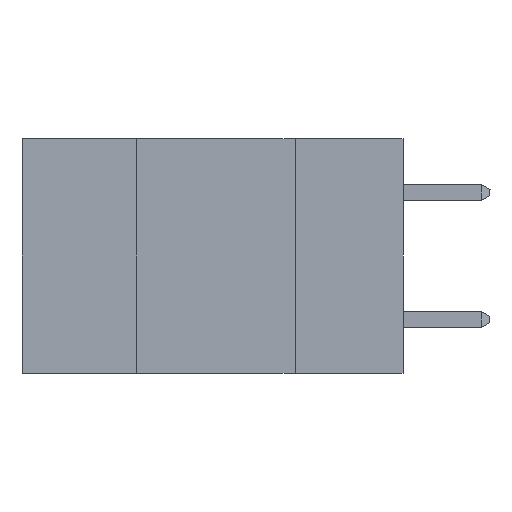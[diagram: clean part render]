
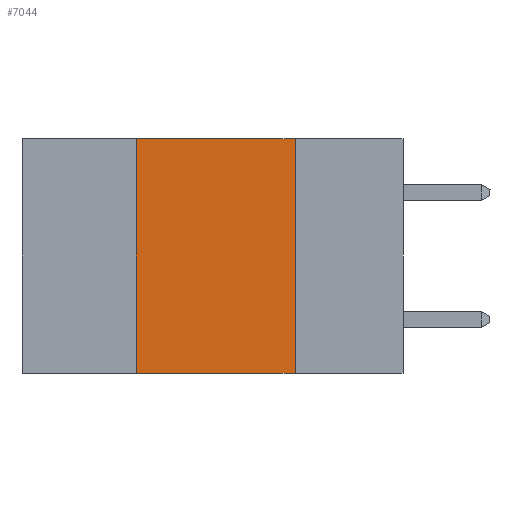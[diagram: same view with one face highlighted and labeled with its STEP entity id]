
A CAD part, left-side view. The second image highlights one B-rep face of the part: STEP entity #7044.
In plain terms, the highlighted planar face has unit normal (-1, 0, 0).
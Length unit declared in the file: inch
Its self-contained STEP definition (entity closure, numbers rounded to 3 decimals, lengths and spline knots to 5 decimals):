
#119 = LINE ( 'NONE', #8788, #1291 ) ;
#154 = CARTESIAN_POINT ( 'NONE',  ( 0., 0.17, -0.37 ) ) ;
#799 = ORIENTED_EDGE ( 'NONE', *, *, #2144, .T. ) ;
#1194 = ORIENTED_EDGE ( 'NONE', *, *, #5678, .F. ) ;
#1291 = VECTOR ( 'NONE', #3387, 39.37008 ) ;
#1504 = LINE ( 'NONE', #10190, #4808 ) ;
#1773 = DIRECTION ( 'NONE',  ( 0., 0., -1. ) ) ;
#2144 = EDGE_CURVE ( 'NONE', #11082, #13219, #7623, .T. ) ;
#2522 = EDGE_LOOP ( 'NONE', ( #8219, #12544, #1194, #799 ) ) ;
#2592 = DIRECTION ( 'NONE',  ( 0., 0., 1. ) ) ;
#2691 = EDGE_CURVE ( 'NONE', #8014, #13219, #1504, .T. ) ;
#3028 = CARTESIAN_POINT ( 'NONE',  ( 0., 0.17, 0. ) ) ;
#3387 = DIRECTION ( 'NONE',  ( 0., -1., 0. ) ) ;
#4664 = CARTESIAN_POINT ( 'NONE',  ( 0., 0.6, 0. ) ) ;
#4808 = VECTOR ( 'NONE', #1773, 39.37008 ) ;
#4813 = LINE ( 'NONE', #5727, #12065 ) ;
#5678 = EDGE_CURVE ( 'NONE', #11082, #12973, #4813, .T. ) ;
#5727 = CARTESIAN_POINT ( 'NONE',  ( 0., 0.42, 0. ) ) ;
#5732 = FACE_OUTER_BOUND ( 'NONE', #2522, .T. ) ;
#6854 = DIRECTION ( 'NONE',  ( 0., -1., 0. ) ) ;
#7044 = ADVANCED_FACE ( 'NONE', ( #5732 ), #10071, .F. ) ;
#7623 = LINE ( 'NONE', #8764, #9974 ) ;
#7770 = CARTESIAN_POINT ( 'NONE',  ( 0., 0.42, 0. ) ) ;
#8014 = VERTEX_POINT ( 'NONE', #3028 ) ;
#8219 = ORIENTED_EDGE ( 'NONE', *, *, #2691, .F. ) ;
#8764 = CARTESIAN_POINT ( 'NONE',  ( 0., 0.6, -0.37 ) ) ;
#8788 = CARTESIAN_POINT ( 'NONE',  ( 0., 0.6, 0. ) ) ;
#9066 = CARTESIAN_POINT ( 'NONE',  ( 0., 0.42, -0.37 ) ) ;
#9974 = VECTOR ( 'NONE', #6854, 39.37008 ) ;
#10071 = PLANE ( 'NONE',  #13772 ) ;
#10138 = DIRECTION ( 'NONE',  ( 1., 0., 0. ) ) ;
#10190 = CARTESIAN_POINT ( 'NONE',  ( 0., 0.17, 0. ) ) ;
#10278 = DIRECTION ( 'NONE',  ( 0., 0., -1. ) ) ;
#10974 = EDGE_CURVE ( 'NONE', #12973, #8014, #119, .T. ) ;
#11082 = VERTEX_POINT ( 'NONE', #9066 ) ;
#12065 = VECTOR ( 'NONE', #2592, 39.37008 ) ;
#12544 = ORIENTED_EDGE ( 'NONE', *, *, #10974, .F. ) ;
#12973 = VERTEX_POINT ( 'NONE', #7770 ) ;
#13219 = VERTEX_POINT ( 'NONE', #154 ) ;
#13772 = AXIS2_PLACEMENT_3D ( 'NONE', #4664, #10138, #10278 ) ;
